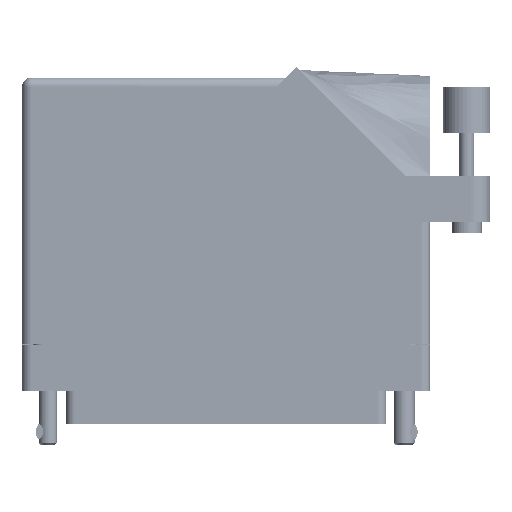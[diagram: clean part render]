
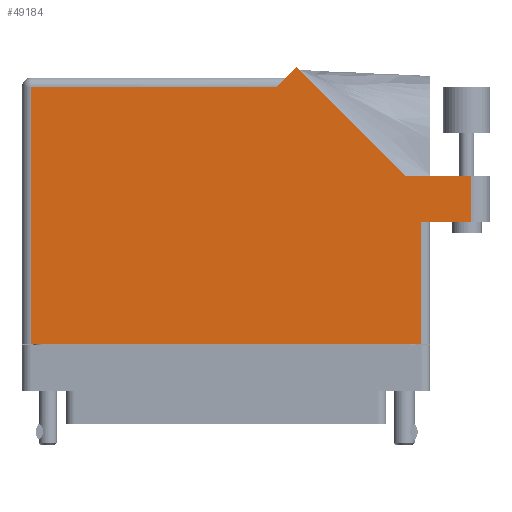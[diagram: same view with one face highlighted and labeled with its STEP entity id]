
A CAD part, front view. The second image highlights one B-rep face of the part: STEP entity #49184.
In plain terms, the highlighted face is planar.
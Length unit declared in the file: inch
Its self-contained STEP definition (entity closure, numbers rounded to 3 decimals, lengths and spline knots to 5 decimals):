
#430 = FACE_OUTER_BOUND ( 'NONE', #40682, .T. ) ;
#1221 = LINE ( 'NONE', #14505, #5937 ) ;
#3458 = CARTESIAN_POINT ( 'NONE',  ( 1.297, 0.715, 0.617 ) ) ;
#5937 = VECTOR ( 'NONE', #34983, 39.37008 ) ;
#7728 = LINE ( 'NONE', #78428, #56437 ) ;
#7858 = ORIENTED_EDGE ( 'NONE', *, *, #19925, .T. ) ;
#8283 = CARTESIAN_POINT ( 'NONE',  ( -1.359, -0.1, 0.617 ) ) ;
#10003 = EDGE_CURVE ( 'NONE', #52689, #47625, #55028, .T. ) ;
#10335 = LINE ( 'NONE', #32893, #81358 ) ;
#11142 = EDGE_CURVE ( 'NONE', #35175, #28094, #59672, .T. ) ;
#11845 = CARTESIAN_POINT ( 'NONE',  ( 1.19342, 1.022, 0.617 ) ) ;
#12668 = CARTESIAN_POINT ( 'NONE',  ( -1.297, -0.1, 0.617 ) ) ;
#14505 = CARTESIAN_POINT ( 'NONE',  ( 1.359, 0.715, 0.617 ) ) ;
#14857 = DIRECTION ( 'NONE',  ( 1., 0., 0. ) ) ;
#15318 = LINE ( 'NONE', #56854, #22559 ) ;
#15643 = ORIENTED_EDGE ( 'NONE', *, *, #10003, .T. ) ;
#17230 = ORIENTED_EDGE ( 'NONE', *, *, #42300, .T. ) ;
#18690 = VECTOR ( 'NONE', #35096, 39.37008 ) ;
#19547 = VERTEX_POINT ( 'NONE', #11845 ) ;
#19925 = EDGE_CURVE ( 'NONE', #38633, #35175, #1221, .T. ) ;
#21442 = CARTESIAN_POINT ( 'NONE',  ( -1.359, 1.613, 0.617 ) ) ;
#22559 = VECTOR ( 'NONE', #71047, 39.37008 ) ;
#27749 = DIRECTION ( 'NONE',  ( 0., 1., 0. ) ) ;
#28094 = VERTEX_POINT ( 'NONE', #69910 ) ;
#29378 = CARTESIAN_POINT ( 'NONE',  ( 1.297, -0.1, 0.617 ) ) ;
#30164 = CARTESIAN_POINT ( 'NONE',  ( 1.759, 1.022, 0.617 ) ) ;
#30408 = LINE ( 'NONE', #30164, #56616 ) ;
#32893 = CARTESIAN_POINT ( 'NONE',  ( 1.297, 0.715, 0.617 ) ) ;
#34824 = CARTESIAN_POINT ( 'NONE',  ( 1.634, 1.022, 0.617 ) ) ;
#34983 = DIRECTION ( 'NONE',  ( 1., 0., 0. ) ) ;
#35096 = DIRECTION ( 'NONE',  ( -1., 0., 0. ) ) ;
#35175 = VERTEX_POINT ( 'NONE', #35198 ) ;
#35198 = CARTESIAN_POINT ( 'NONE',  ( 1.634, 0.715, 0.617 ) ) ;
#35836 = VECTOR ( 'NONE', #56002, 39.37008 ) ;
#37801 = ORIENTED_EDGE ( 'NONE', *, *, #56846, .T. ) ;
#38257 = PLANE ( 'NONE',  #49237 ) ;
#38633 = VERTEX_POINT ( 'NONE', #3458 ) ;
#39458 = ORIENTED_EDGE ( 'NONE', *, *, #77810, .T. ) ;
#40599 = ORIENTED_EDGE ( 'NONE', *, *, #41347, .T. ) ;
#40682 = EDGE_LOOP ( 'NONE', ( #7858, #59293, #83374, #37801, #39458, #77921, #17230, #15643, #40599 ) ) ;
#41347 = EDGE_CURVE ( 'NONE', #47625, #38633, #10335, .T. ) ;
#42300 = EDGE_CURVE ( 'NONE', #43480, #52689, #15318, .T. ) ;
#43186 = DIRECTION ( 'NONE',  ( -1., 0., 0. ) ) ;
#43480 = VERTEX_POINT ( 'NONE', #55000 ) ;
#44728 = DIRECTION ( 'NONE',  ( -1., 0., 0. ) ) ;
#47625 = VERTEX_POINT ( 'NONE', #29378 ) ;
#49184 = ADVANCED_FACE ( 'NONE', ( #430 ), #38257, .F. ) ;
#49237 = AXIS2_PLACEMENT_3D ( 'NONE', #70287, #82767, #44728 ) ;
#51732 = DIRECTION ( 'NONE',  ( -0.707, -0.707, 0. ) ) ;
#52689 = VERTEX_POINT ( 'NONE', #12668 ) ;
#54064 = VERTEX_POINT ( 'NONE', #71654 ) ;
#55000 = CARTESIAN_POINT ( 'NONE',  ( -1.297, 1.613, 0.617 ) ) ;
#55028 = LINE ( 'NONE', #8283, #70253 ) ;
#56002 = DIRECTION ( 'NONE',  ( -0.707, 0.707, 0. ) ) ;
#56437 = VECTOR ( 'NONE', #51732, 39.37008 ) ;
#56616 = VECTOR ( 'NONE', #43186, 39.37008 ) ;
#56846 = EDGE_CURVE ( 'NONE', #19547, #83272, #65238, .T. ) ;
#56854 = CARTESIAN_POINT ( 'NONE',  ( -1.297, -0.1, 0.617 ) ) ;
#59293 = ORIENTED_EDGE ( 'NONE', *, *, #11142, .T. ) ;
#59672 = LINE ( 'NONE', #34824, #72881 ) ;
#60035 = EDGE_CURVE ( 'NONE', #28094, #19547, #30408, .T. ) ;
#65238 = LINE ( 'NONE', #82366, #35836 ) ;
#69910 = CARTESIAN_POINT ( 'NONE',  ( 1.634, 1.022, 0.617 ) ) ;
#70253 = VECTOR ( 'NONE', #14857, 39.37008 ) ;
#70287 = CARTESIAN_POINT ( 'NONE',  ( -1.359, 1.675, 0.617 ) ) ;
#71047 = DIRECTION ( 'NONE',  ( 0., -1., 0. ) ) ;
#71654 = CARTESIAN_POINT ( 'NONE',  ( 0.337, 1.613, 0.617 ) ) ;
#71989 = EDGE_CURVE ( 'NONE', #54064, #43480, #75535, .T. ) ;
#72881 = VECTOR ( 'NONE', #27749, 39.37008 ) ;
#75535 = LINE ( 'NONE', #21442, #18690 ) ;
#77810 = EDGE_CURVE ( 'NONE', #83272, #54064, #7728, .T. ) ;
#77921 = ORIENTED_EDGE ( 'NONE', *, *, #71989, .T. ) ;
#78199 = DIRECTION ( 'NONE',  ( 0., 1., 0. ) ) ;
#78428 = CARTESIAN_POINT ( 'NONE',  ( 0.399, 1.675, 0.617 ) ) ;
#81358 = VECTOR ( 'NONE', #78199, 39.37008 ) ;
#81988 = CARTESIAN_POINT ( 'NONE',  ( 0.46971, 1.74571, 0.617 ) ) ;
#82366 = CARTESIAN_POINT ( 'NONE',  ( 1.19342, 1.022, 0.617 ) ) ;
#82767 = DIRECTION ( 'NONE',  ( 0., 0., -1. ) ) ;
#83272 = VERTEX_POINT ( 'NONE', #81988 ) ;
#83374 = ORIENTED_EDGE ( 'NONE', *, *, #60035, .T. ) ;
